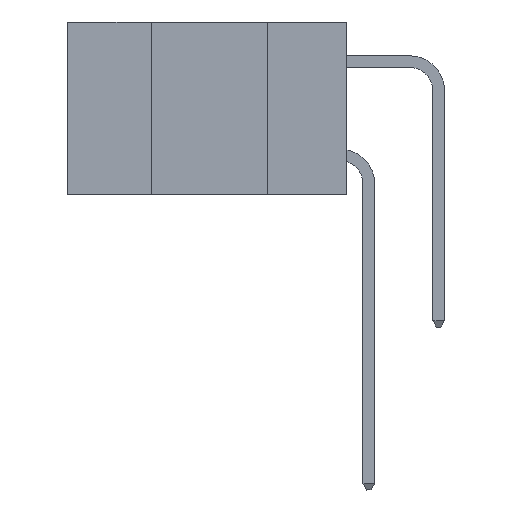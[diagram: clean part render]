
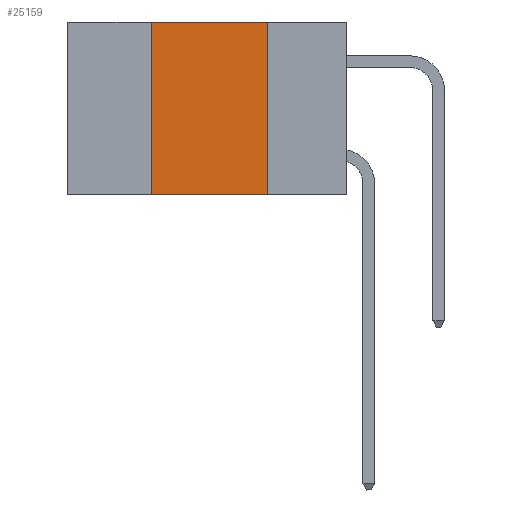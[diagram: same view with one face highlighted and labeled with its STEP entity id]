
A CAD part, left-side view. The second image highlights one B-rep face of the part: STEP entity #25159.
In plain terms, the highlighted planar face has unit normal (-1, 0, 0).
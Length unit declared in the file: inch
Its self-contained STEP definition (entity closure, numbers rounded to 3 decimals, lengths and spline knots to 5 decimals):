
#680 = VERTEX_POINT ( 'NONE', #29377 ) ;
#1067 = ORIENTED_EDGE ( 'NONE', *, *, #19903, .F. ) ;
#1239 = VERTEX_POINT ( 'NONE', #8583 ) ;
#1441 = VECTOR ( 'NONE', #15641, 39.37008 ) ;
#1722 = ORIENTED_EDGE ( 'NONE', *, *, #14913, .F. ) ;
#2364 = VECTOR ( 'NONE', #12970, 39.37008 ) ;
#3393 = CARTESIAN_POINT ( 'NONE',  ( 0., 0.17, 0. ) ) ;
#4674 = EDGE_CURVE ( 'NONE', #680, #1239, #14633, .T. ) ;
#5552 = LINE ( 'NONE', #11197, #26594 ) ;
#5854 = CARTESIAN_POINT ( 'NONE',  ( 0., 0.6, 0. ) ) ;
#8583 = CARTESIAN_POINT ( 'NONE',  ( 0., 0.17, -0.37 ) ) ;
#8697 = LINE ( 'NONE', #5854, #2364 ) ;
#8858 = PLANE ( 'NONE',  #17763 ) ;
#10128 = DIRECTION ( 'NONE',  ( 0., 0., -1. ) ) ;
#10493 = CARTESIAN_POINT ( 'NONE',  ( 0., 0.6, -0.37 ) ) ;
#10582 = VERTEX_POINT ( 'NONE', #22563 ) ;
#11197 = CARTESIAN_POINT ( 'NONE',  ( 0., 0.17, 0. ) ) ;
#11717 = VECTOR ( 'NONE', #24459, 39.37008 ) ;
#12970 = DIRECTION ( 'NONE',  ( 0., -1., 0. ) ) ;
#14633 = LINE ( 'NONE', #10493, #11717 ) ;
#14913 = EDGE_CURVE ( 'NONE', #17115, #1239, #5552, .T. ) ;
#15641 = DIRECTION ( 'NONE',  ( 0., 0., 1. ) ) ;
#16016 = EDGE_CURVE ( 'NONE', #10582, #17115, #8697, .T. ) ;
#16164 = DIRECTION ( 'NONE',  ( 1., 0., 0. ) ) ;
#16275 = ORIENTED_EDGE ( 'NONE', *, *, #4674, .T. ) ;
#16324 = CARTESIAN_POINT ( 'NONE',  ( 0., 0.6, 0. ) ) ;
#16547 = EDGE_LOOP ( 'NONE', ( #1722, #18471, #1067, #16275 ) ) ;
#17115 = VERTEX_POINT ( 'NONE', #3393 ) ;
#17763 = AXIS2_PLACEMENT_3D ( 'NONE', #16324, #16164, #23760 ) ;
#18013 = CARTESIAN_POINT ( 'NONE',  ( 0., 0.42, 0. ) ) ;
#18471 = ORIENTED_EDGE ( 'NONE', *, *, #16016, .F. ) ;
#19903 = EDGE_CURVE ( 'NONE', #680, #10582, #20398, .T. ) ;
#20398 = LINE ( 'NONE', #18013, #1441 ) ;
#22563 = CARTESIAN_POINT ( 'NONE',  ( 0., 0.42, 0. ) ) ;
#23760 = DIRECTION ( 'NONE',  ( 0., 0., -1. ) ) ;
#24459 = DIRECTION ( 'NONE',  ( 0., -1., 0. ) ) ;
#25159 = ADVANCED_FACE ( 'NONE', ( #26286 ), #8858, .F. ) ;
#26286 = FACE_OUTER_BOUND ( 'NONE', #16547, .T. ) ;
#26594 = VECTOR ( 'NONE', #10128, 39.37008 ) ;
#29377 = CARTESIAN_POINT ( 'NONE',  ( 0., 0.42, -0.37 ) ) ;
